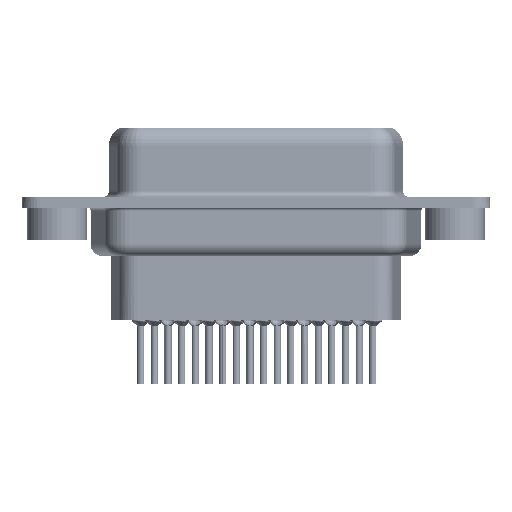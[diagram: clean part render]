
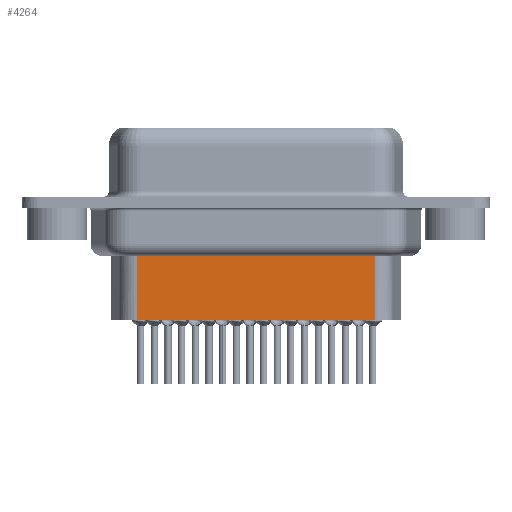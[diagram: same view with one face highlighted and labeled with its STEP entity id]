
A CAD part, front view. The second image highlights one B-rep face of the part: STEP entity #4264.
In plain terms, the highlighted planar face has unit normal (0, -1, 0).
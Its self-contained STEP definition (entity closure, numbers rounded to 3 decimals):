
#662 = DIRECTION ( 'NONE',  ( 0., -1., 0. ) ) ;
#1141 = DIRECTION ( 'NONE',  ( 1., 0., 0. ) ) ;
#1733 = CARTESIAN_POINT ( 'NONE',  ( 6.691, -3.5, -9.85 ) ) ;
#2772 = ORIENTED_EDGE ( 'NONE', *, *, #20583, .F. ) ;
#4264 = ADVANCED_FACE ( 'NONE', ( #23674 ), #18373, .T. ) ;
#4805 = CARTESIAN_POINT ( 'NONE',  ( 6.691, -3.5, -3.1 ) ) ;
#5916 = AXIS2_PLACEMENT_3D ( 'NONE', #6275, #662, #1141 ) ;
#6275 = CARTESIAN_POINT ( 'NONE',  ( 6.691, -3.5, -3.1 ) ) ;
#6978 = LINE ( 'NONE', #4805, #13293 ) ;
#7867 = CARTESIAN_POINT ( 'NONE',  ( 26.629, -3.5, -4.097 ) ) ;
#8263 = CARTESIAN_POINT ( 'NONE',  ( 6.691, -3.5, -9.85 ) ) ;
#8308 = ORIENTED_EDGE ( 'NONE', *, *, #13961, .T. ) ;
#8407 = EDGE_LOOP ( 'NONE', ( #15975, #14334, #8308, #2772 ) ) ;
#9416 = VECTOR ( 'NONE', #15653, 1000. ) ;
#12596 = DIRECTION ( 'NONE',  ( 0., 0., -1. ) ) ;
#13175 = DIRECTION ( 'NONE',  ( -1., 0., 0. ) ) ;
#13195 = EDGE_CURVE ( 'NONE', #29549, #32037, #28580, .T. ) ;
#13293 = VECTOR ( 'NONE', #12596, 1000. ) ;
#13961 = EDGE_CURVE ( 'NONE', #32037, #20224, #6978, .T. ) ;
#13983 = DIRECTION ( 'NONE',  ( -1., 0., 0. ) ) ;
#14334 = ORIENTED_EDGE ( 'NONE', *, *, #13195, .T. ) ;
#15653 = DIRECTION ( 'NONE',  ( 0., 0., -1. ) ) ;
#15975 = ORIENTED_EDGE ( 'NONE', *, *, #32744, .F. ) ;
#18373 = PLANE ( 'NONE',  #5916 ) ;
#18998 = VERTEX_POINT ( 'NONE', #19882 ) ;
#19882 = CARTESIAN_POINT ( 'NONE',  ( 26.629, -3.5, -9.85 ) ) ;
#20224 = VERTEX_POINT ( 'NONE', #8263 ) ;
#20583 = EDGE_CURVE ( 'NONE', #18998, #20224, #24445, .T. ) ;
#20780 = CARTESIAN_POINT ( 'NONE',  ( 26.629, -3.5, -3.1 ) ) ;
#22715 = CARTESIAN_POINT ( 'NONE',  ( 6.691, -3.5, -4.097 ) ) ;
#23674 = FACE_OUTER_BOUND ( 'NONE', #8407, .T. ) ;
#24445 = LINE ( 'NONE', #1733, #27844 ) ;
#26273 = CARTESIAN_POINT ( 'NONE',  ( 6.444, -3.5, -4.097 ) ) ;
#27844 = VECTOR ( 'NONE', #13983, 1000. ) ;
#28238 = LINE ( 'NONE', #20780, #9416 ) ;
#28580 = LINE ( 'NONE', #26273, #31266 ) ;
#29549 = VERTEX_POINT ( 'NONE', #7867 ) ;
#31266 = VECTOR ( 'NONE', #13175, 1000. ) ;
#32037 = VERTEX_POINT ( 'NONE', #22715 ) ;
#32744 = EDGE_CURVE ( 'NONE', #29549, #18998, #28238, .T. ) ;
